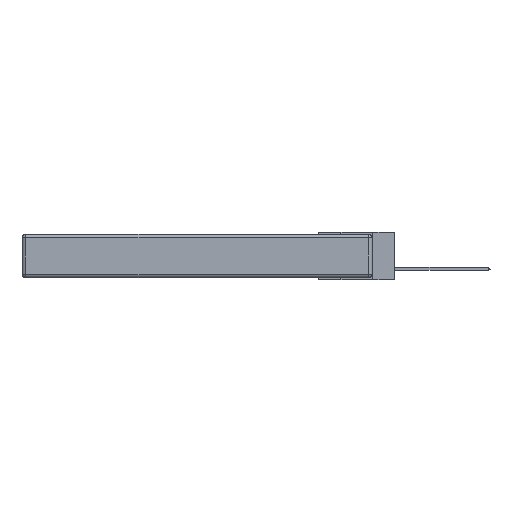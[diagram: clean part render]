
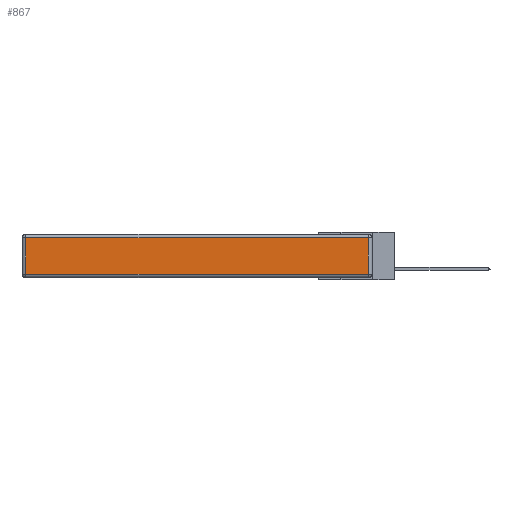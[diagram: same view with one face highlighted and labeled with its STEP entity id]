
A CAD part, left-side view. The second image highlights one B-rep face of the part: STEP entity #867.
In plain terms, the highlighted planar face has unit normal (-1, 0, 0).
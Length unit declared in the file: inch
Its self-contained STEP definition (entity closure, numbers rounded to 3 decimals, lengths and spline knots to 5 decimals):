
#674 = VECTOR ( 'NONE', #4527, 39.37008 ) ;
#867 = ADVANCED_FACE ( 'NONE', ( #15439 ), #19491, .T. ) ;
#1240 = DIRECTION ( 'NONE',  ( 0., -1., 0. ) ) ;
#1965 = VECTOR ( 'NONE', #22263, 39.37008 ) ;
#3059 = ORIENTED_EDGE ( 'NONE', *, *, #12350, .T. ) ;
#3921 = DIRECTION ( 'NONE',  ( -1., 0., 0. ) ) ;
#4305 = CARTESIAN_POINT ( 'NONE',  ( 0., 0.03, -0.03 ) ) ;
#4311 = EDGE_LOOP ( 'NONE', ( #11152, #3059, #21054, #14780 ) ) ;
#4527 = DIRECTION ( 'NONE',  ( 0., 0., 1. ) ) ;
#5558 = VERTEX_POINT ( 'NONE', #20007 ) ;
#6541 = EDGE_CURVE ( 'NONE', #16642, #16254, #9007, .T. ) ;
#7424 = CARTESIAN_POINT ( 'NONE',  ( 0., 0., -0.343 ) ) ;
#7557 = LINE ( 'NONE', #15043, #8641 ) ;
#8157 = CARTESIAN_POINT ( 'NONE',  ( 0., 2.72, -0.313 ) ) ;
#8296 = LINE ( 'NONE', #20837, #14255 ) ;
#8641 = VECTOR ( 'NONE', #1240, 39.37008 ) ;
#9007 = LINE ( 'NONE', #10123, #1965 ) ;
#10123 = CARTESIAN_POINT ( 'NONE',  ( 0., 2.72, -0.343 ) ) ;
#11152 = ORIENTED_EDGE ( 'NONE', *, *, #16810, .T. ) ;
#12350 = EDGE_CURVE ( 'NONE', #5558, #21972, #21318, .T. ) ;
#12539 = CARTESIAN_POINT ( 'NONE',  ( 0., 2.72, -0.03 ) ) ;
#12638 = DIRECTION ( 'NONE',  ( 0., 0., 1. ) ) ;
#13929 = DIRECTION ( 'NONE',  ( 0., 1., 0. ) ) ;
#14255 = VECTOR ( 'NONE', #13929, 39.37008 ) ;
#14780 = ORIENTED_EDGE ( 'NONE', *, *, #6541, .T. ) ;
#15043 = CARTESIAN_POINT ( 'NONE',  ( 0., 0., -0.313 ) ) ;
#15439 = FACE_OUTER_BOUND ( 'NONE', #4311, .T. ) ;
#16254 = VERTEX_POINT ( 'NONE', #8157 ) ;
#16642 = VERTEX_POINT ( 'NONE', #12539 ) ;
#16810 = EDGE_CURVE ( 'NONE', #16254, #5558, #7557, .T. ) ;
#18140 = CARTESIAN_POINT ( 'NONE',  ( 0., 0.03, -0.343 ) ) ;
#18785 = AXIS2_PLACEMENT_3D ( 'NONE', #7424, #3921, #12638 ) ;
#19394 = EDGE_CURVE ( 'NONE', #21972, #16642, #8296, .T. ) ;
#19491 = PLANE ( 'NONE',  #18785 ) ;
#20007 = CARTESIAN_POINT ( 'NONE',  ( 0., 0.03, -0.313 ) ) ;
#20837 = CARTESIAN_POINT ( 'NONE',  ( 0., 2.75, -0.03 ) ) ;
#21054 = ORIENTED_EDGE ( 'NONE', *, *, #19394, .T. ) ;
#21318 = LINE ( 'NONE', #18140, #674 ) ;
#21972 = VERTEX_POINT ( 'NONE', #4305 ) ;
#22263 = DIRECTION ( 'NONE',  ( 0., 0., -1. ) ) ;
